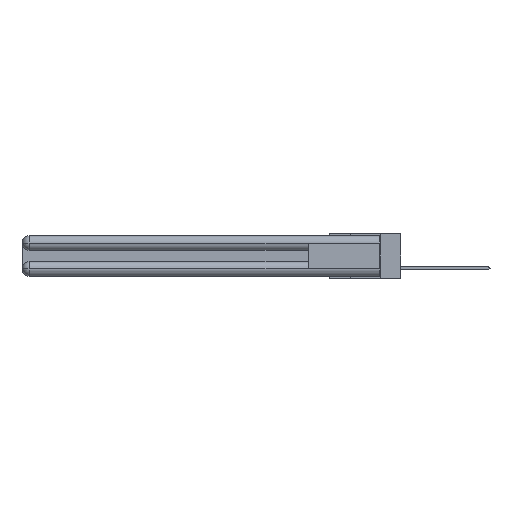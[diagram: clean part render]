
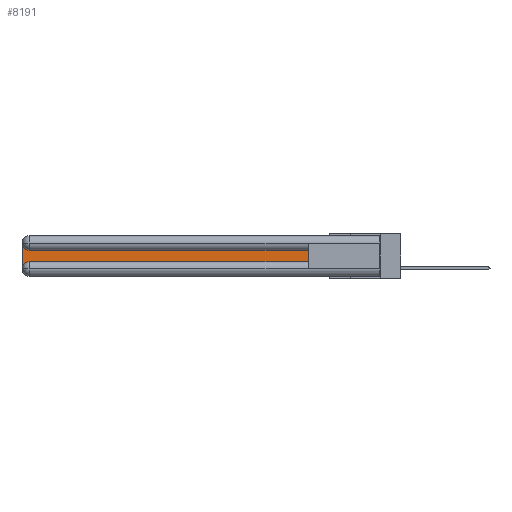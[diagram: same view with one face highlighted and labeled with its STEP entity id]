
A CAD part, left-side view. The second image highlights one B-rep face of the part: STEP entity #8191.
In plain terms, the highlighted planar face has unit normal (-1, 0, 0).
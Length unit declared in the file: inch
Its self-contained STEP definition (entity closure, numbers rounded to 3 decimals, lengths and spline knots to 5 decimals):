
#1338 = ORIENTED_EDGE ( 'NONE', *, *, #16143, .T. ) ;
#1460 = VECTOR ( 'NONE', #10044, 39.37008 ) ;
#2661 = CARTESIAN_POINT ( 'NONE',  ( 0.075, 0.6, -0.1225 ) ) ;
#2710 = DIRECTION ( 'NONE',  ( 1., 0., 0. ) ) ;
#2806 = AXIS2_PLACEMENT_3D ( 'NONE', #8189, #27310, #26948 ) ;
#2864 = DIRECTION ( 'NONE',  ( 0., 1., 0. ) ) ;
#3630 = CARTESIAN_POINT ( 'NONE',  ( 0.075, 2.94, -0.1225 ) ) ;
#3857 = DIRECTION ( 'NONE',  ( 0., 0., 1. ) ) ;
#5146 = DIRECTION ( 'NONE',  ( 0., 0., -1. ) ) ;
#5651 = EDGE_LOOP ( 'NONE', ( #1338, #15458, #23314, #23200, #25639, #16645 ) ) ;
#5796 = VERTEX_POINT ( 'NONE', #26011 ) ;
#5817 = CARTESIAN_POINT ( 'NONE',  ( 0.075, 3., -0.2175 ) ) ;
#6744 = CARTESIAN_POINT ( 'NONE',  ( 0.075, 0.6, -0.1225 ) ) ;
#8184 = AXIS2_PLACEMENT_3D ( 'NONE', #21531, #2710, #5146 ) ;
#8189 = CARTESIAN_POINT ( 'NONE',  ( 0.075, 2.94, -0.0625 ) ) ;
#8191 = ADVANCED_FACE ( 'NONE', ( #13243 ), #34505, .F. ) ;
#10044 = DIRECTION ( 'NONE',  ( 0., 0., -1. ) ) ;
#10186 = CARTESIAN_POINT ( 'NONE',  ( 0.075, 0.6, -0.2175 ) ) ;
#10372 = DIRECTION ( 'NONE',  ( 0., 0., -1. ) ) ;
#10937 = CARTESIAN_POINT ( 'NONE',  ( 0.075, 0.6, -0.2175 ) ) ;
#12103 = LINE ( 'NONE', #10186, #23003 ) ;
#12377 = EDGE_CURVE ( 'NONE', #5796, #33431, #12103, .T. ) ;
#12960 = CIRCLE ( 'NONE', #2806, 0.06 ) ;
#13243 = FACE_OUTER_BOUND ( 'NONE', #5651, .T. ) ;
#13278 = EDGE_CURVE ( 'NONE', #19684, #32606, #12960, .T. ) ;
#14724 = CARTESIAN_POINT ( 'NONE',  ( 0.075, 0.6, -0.2175 ) ) ;
#15458 = ORIENTED_EDGE ( 'NONE', *, *, #13278, .T. ) ;
#15896 = CARTESIAN_POINT ( 'NONE',  ( 0.075, 2.94, -0.2775 ) ) ;
#16143 = EDGE_CURVE ( 'NONE', #27367, #19684, #34129, .T. ) ;
#16645 = ORIENTED_EDGE ( 'NONE', *, *, #31395, .T. ) ;
#19684 = VERTEX_POINT ( 'NONE', #3630 ) ;
#19788 = EDGE_CURVE ( 'NONE', #20453, #5796, #27320, .T. ) ;
#20453 = VERTEX_POINT ( 'NONE', #23764 ) ;
#20979 = DIRECTION ( 'NONE',  ( 0., -1., 0. ) ) ;
#21531 = CARTESIAN_POINT ( 'NONE',  ( 0.075, 3., -0.1225 ) ) ;
#22095 = VECTOR ( 'NONE', #3857, 39.37008 ) ;
#23003 = VECTOR ( 'NONE', #20979, 39.37008 ) ;
#23200 = ORIENTED_EDGE ( 'NONE', *, *, #19788, .T. ) ;
#23314 = ORIENTED_EDGE ( 'NONE', *, *, #33141, .T. ) ;
#23764 = CARTESIAN_POINT ( 'NONE',  ( 0.075, 3., -0.2775 ) ) ;
#25634 = AXIS2_PLACEMENT_3D ( 'NONE', #15896, #34618, #10372 ) ;
#25639 = ORIENTED_EDGE ( 'NONE', *, *, #12377, .T. ) ;
#25705 = LINE ( 'NONE', #5817, #1460 ) ;
#26011 = CARTESIAN_POINT ( 'NONE',  ( 0.075, 2.94, -0.2175 ) ) ;
#26948 = DIRECTION ( 'NONE',  ( 0., 0., -1. ) ) ;
#27310 = DIRECTION ( 'NONE',  ( 1., 0., 0. ) ) ;
#27320 = CIRCLE ( 'NONE', #25634, 0.06 ) ;
#27367 = VERTEX_POINT ( 'NONE', #2661 ) ;
#30863 = LINE ( 'NONE', #14724, #22095 ) ;
#31395 = EDGE_CURVE ( 'NONE', #33431, #27367, #30863, .T. ) ;
#32606 = VERTEX_POINT ( 'NONE', #33232 ) ;
#33141 = EDGE_CURVE ( 'NONE', #32606, #20453, #25705, .T. ) ;
#33232 = CARTESIAN_POINT ( 'NONE',  ( 0.075, 3., -0.0625 ) ) ;
#33431 = VERTEX_POINT ( 'NONE', #10937 ) ;
#34129 = LINE ( 'NONE', #6744, #34168 ) ;
#34168 = VECTOR ( 'NONE', #2864, 39.37008 ) ;
#34505 = PLANE ( 'NONE',  #8184 ) ;
#34618 = DIRECTION ( 'NONE',  ( 1., 0., 0. ) ) ;
